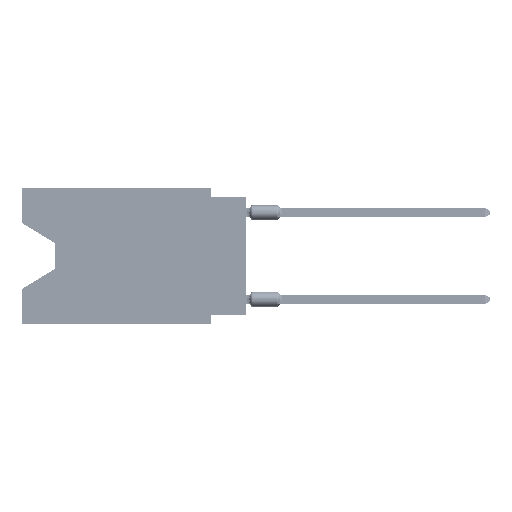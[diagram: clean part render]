
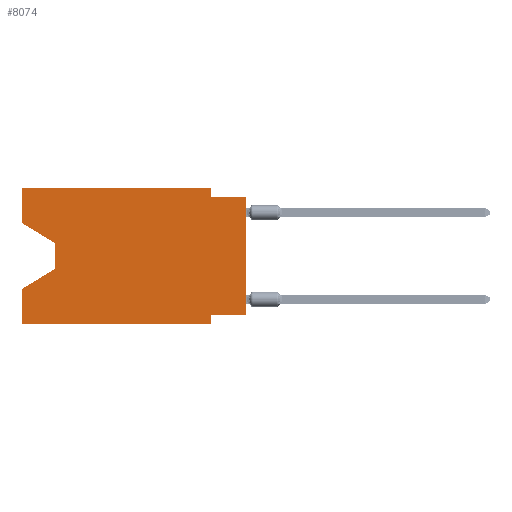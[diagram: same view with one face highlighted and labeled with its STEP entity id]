
A CAD part, left-side view. The second image highlights one B-rep face of the part: STEP entity #8074.
In plain terms, the highlighted planar face has unit normal (-1, 0, 0).
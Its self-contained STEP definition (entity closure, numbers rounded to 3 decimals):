
#1159 = LINE ( 'NONE', #34626, #59074 ) ;
#1394 = CARTESIAN_POINT ( 'NONE',  ( 0., 2.54, -9.906 ) ) ;
#1523 = FACE_OUTER_BOUND ( 'NONE', #3938, .T. ) ;
#2123 = CARTESIAN_POINT ( 'NONE',  ( 0., 2.54, 0. ) ) ;
#2851 = VECTOR ( 'NONE', #4424, 1000. ) ;
#2863 = ORIENTED_EDGE ( 'NONE', *, *, #10819, .F. ) ;
#2867 = CARTESIAN_POINT ( 'NONE',  ( 0., 16.383, 0. ) ) ;
#3063 = ORIENTED_EDGE ( 'NONE', *, *, #20691, .T. ) ;
#3105 = VERTEX_POINT ( 'NONE', #59620 ) ;
#3376 = CARTESIAN_POINT ( 'NONE',  ( 0., 16.383, -2.546 ) ) ;
#3691 = CARTESIAN_POINT ( 'NONE',  ( 0., 0., -0.635 ) ) ;
#3742 = CARTESIAN_POINT ( 'NONE',  ( 0., 13.97, -4.013 ) ) ;
#3938 = EDGE_LOOP ( 'NONE', ( #64744, #59854, #3063, #28875, #27565, #47178, #2863, #46202, #27620, #20472, #58331, #59288 ) ) ;
#4167 = EDGE_CURVE ( 'NONE', #35852, #37192, #52147, .T. ) ;
#4424 = DIRECTION ( 'NONE',  ( 0., -1., 0. ) ) ;
#5179 = LINE ( 'NONE', #43645, #64525 ) ;
#6237 = EDGE_CURVE ( 'NONE', #68892, #48642, #5179, .T. ) ;
#6455 = VECTOR ( 'NONE', #59240, 1000. ) ;
#6473 = VECTOR ( 'NONE', #36753, 1000. ) ;
#6876 = VERTEX_POINT ( 'NONE', #34892 ) ;
#7638 = CARTESIAN_POINT ( 'NONE',  ( 0., 2.54, -0.635 ) ) ;
#8074 = ADVANCED_FACE ( 'NONE', ( #1523 ), #23254, .F. ) ;
#8159 = EDGE_CURVE ( 'NONE', #39232, #6876, #31767, .T. ) ;
#8927 = CARTESIAN_POINT ( 'NONE',  ( 0., 16.383, -2.546 ) ) ;
#10819 = EDGE_CURVE ( 'NONE', #48529, #58875, #1159, .T. ) ;
#11024 = DIRECTION ( 'NONE',  ( 0., 0., -1. ) ) ;
#13255 = AXIS2_PLACEMENT_3D ( 'NONE', #44977, #29632, #66717 ) ;
#16393 = LINE ( 'NONE', #37093, #42469 ) ;
#16508 = EDGE_CURVE ( 'NONE', #26429, #39232, #46474, .T. ) ;
#16798 = LINE ( 'NONE', #22510, #6455 ) ;
#17930 = VECTOR ( 'NONE', #49221, 1000. ) ;
#20472 = ORIENTED_EDGE ( 'NONE', *, *, #20558, .F. ) ;
#20558 = EDGE_CURVE ( 'NONE', #48642, #49145, #25743, .T. ) ;
#20691 = EDGE_CURVE ( 'NONE', #6876, #3105, #49572, .T. ) ;
#20945 = VECTOR ( 'NONE', #59233, 1000. ) ;
#21339 = CARTESIAN_POINT ( 'NONE',  ( 0., 2.54, -9.906 ) ) ;
#22331 = EDGE_CURVE ( 'NONE', #58875, #37192, #27771, .T. ) ;
#22510 = CARTESIAN_POINT ( 'NONE',  ( 0., 0., 0. ) ) ;
#23254 = PLANE ( 'NONE',  #13255 ) ;
#24906 = EDGE_CURVE ( 'NONE', #49145, #31231, #32847, .T. ) ;
#25096 = DIRECTION ( 'NONE',  ( 0., -0.855, -0.519 ) ) ;
#25743 = LINE ( 'NONE', #37484, #20945 ) ;
#26429 = VERTEX_POINT ( 'NONE', #8927 ) ;
#27565 = ORIENTED_EDGE ( 'NONE', *, *, #4167, .T. ) ;
#27591 = LINE ( 'NONE', #2867, #42020 ) ;
#27620 = ORIENTED_EDGE ( 'NONE', *, *, #24906, .F. ) ;
#27771 = LINE ( 'NONE', #1394, #33677 ) ;
#28192 = CARTESIAN_POINT ( 'NONE',  ( 0., 13.97, -5.893 ) ) ;
#28291 = DIRECTION ( 'NONE',  ( 0., 0., 1. ) ) ;
#28408 = EDGE_CURVE ( 'NONE', #48529, #31231, #16798, .T. ) ;
#28875 = ORIENTED_EDGE ( 'NONE', *, *, #63798, .F. ) ;
#29632 = DIRECTION ( 'NONE',  ( 1., 0., 0. ) ) ;
#31231 = VERTEX_POINT ( 'NONE', #3691 ) ;
#31767 = LINE ( 'NONE', #36044, #6473 ) ;
#32807 = DIRECTION ( 'NONE',  ( 0., 0., 1. ) ) ;
#32808 = CARTESIAN_POINT ( 'NONE',  ( 0., 0., -9.271 ) ) ;
#32847 = LINE ( 'NONE', #49569, #17930 ) ;
#33677 = VECTOR ( 'NONE', #11024, 1000. ) ;
#33929 = CARTESIAN_POINT ( 'NONE',  ( 0., 2.54, -9.271 ) ) ;
#34626 = CARTESIAN_POINT ( 'NONE',  ( 0., 0., -9.271 ) ) ;
#34892 = CARTESIAN_POINT ( 'NONE',  ( 0., 13.97, -5.893 ) ) ;
#35852 = VERTEX_POINT ( 'NONE', #37313 ) ;
#36044 = CARTESIAN_POINT ( 'NONE',  ( 0., 13.97, -4.013 ) ) ;
#36753 = DIRECTION ( 'NONE',  ( 0., 0., -1. ) ) ;
#37093 = CARTESIAN_POINT ( 'NONE',  ( 0., 16.383, 0. ) ) ;
#37192 = VERTEX_POINT ( 'NONE', #21339 ) ;
#37313 = CARTESIAN_POINT ( 'NONE',  ( 0., 16.383, -9.906 ) ) ;
#37484 = CARTESIAN_POINT ( 'NONE',  ( 0., 2.54, 0. ) ) ;
#38294 = DIRECTION ( 'NONE',  ( 0., -1., 0. ) ) ;
#39232 = VERTEX_POINT ( 'NONE', #3742 ) ;
#42020 = VECTOR ( 'NONE', #28291, 1000. ) ;
#42469 = VECTOR ( 'NONE', #32807, 1000. ) ;
#43645 = CARTESIAN_POINT ( 'NONE',  ( 0., 16.383, 0. ) ) ;
#44977 = CARTESIAN_POINT ( 'NONE',  ( 0., 16.383, 0. ) ) ;
#46202 = ORIENTED_EDGE ( 'NONE', *, *, #28408, .T. ) ;
#46474 = LINE ( 'NONE', #3376, #61564 ) ;
#47178 = ORIENTED_EDGE ( 'NONE', *, *, #22331, .F. ) ;
#48225 = CARTESIAN_POINT ( 'NONE',  ( 0., 16.383, -9.906 ) ) ;
#48529 = VERTEX_POINT ( 'NONE', #32808 ) ;
#48642 = VERTEX_POINT ( 'NONE', #2123 ) ;
#49145 = VERTEX_POINT ( 'NONE', #7638 ) ;
#49221 = DIRECTION ( 'NONE',  ( 0., -1., 0. ) ) ;
#49569 = CARTESIAN_POINT ( 'NONE',  ( 0., 0., -0.635 ) ) ;
#49572 = LINE ( 'NONE', #28192, #53993 ) ;
#50990 = DIRECTION ( 'NONE',  ( 0., 1., 0. ) ) ;
#52147 = LINE ( 'NONE', #48225, #2851 ) ;
#53993 = VECTOR ( 'NONE', #60976, 1000. ) ;
#58331 = ORIENTED_EDGE ( 'NONE', *, *, #6237, .F. ) ;
#58875 = VERTEX_POINT ( 'NONE', #33929 ) ;
#59074 = VECTOR ( 'NONE', #50990, 1000. ) ;
#59233 = DIRECTION ( 'NONE',  ( 0., 0., -1. ) ) ;
#59240 = DIRECTION ( 'NONE',  ( 0., 0., 1. ) ) ;
#59288 = ORIENTED_EDGE ( 'NONE', *, *, #59741, .F. ) ;
#59620 = CARTESIAN_POINT ( 'NONE',  ( 0., 16.383, -7.36 ) ) ;
#59741 = EDGE_CURVE ( 'NONE', #26429, #68892, #27591, .T. ) ;
#59854 = ORIENTED_EDGE ( 'NONE', *, *, #8159, .T. ) ;
#60976 = DIRECTION ( 'NONE',  ( 0., 0.855, -0.519 ) ) ;
#61564 = VECTOR ( 'NONE', #25096, 1000. ) ;
#63798 = EDGE_CURVE ( 'NONE', #35852, #3105, #16393, .T. ) ;
#64279 = CARTESIAN_POINT ( 'NONE',  ( 0., 16.383, 0. ) ) ;
#64525 = VECTOR ( 'NONE', #38294, 1000. ) ;
#64744 = ORIENTED_EDGE ( 'NONE', *, *, #16508, .T. ) ;
#66717 = DIRECTION ( 'NONE',  ( 0., 0., -1. ) ) ;
#68892 = VERTEX_POINT ( 'NONE', #64279 ) ;
